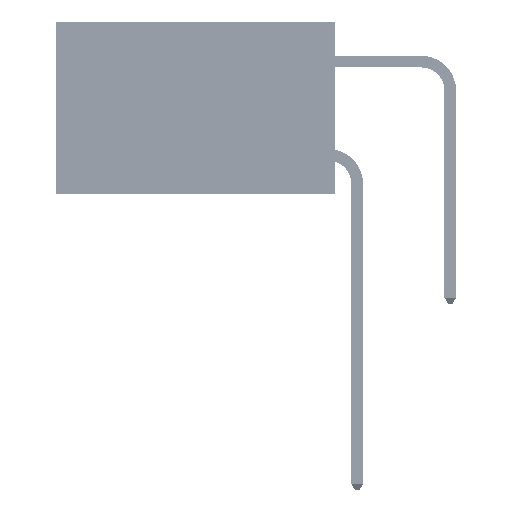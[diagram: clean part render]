
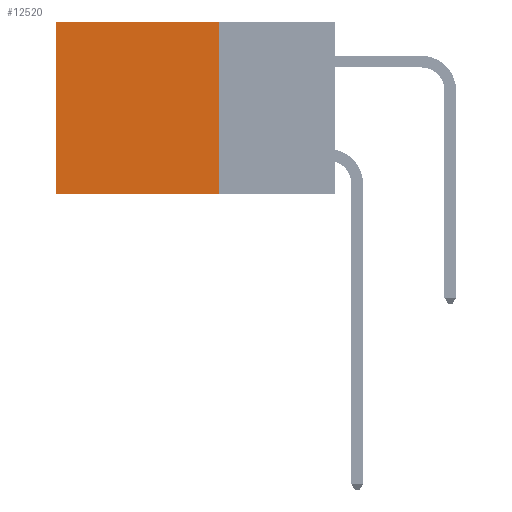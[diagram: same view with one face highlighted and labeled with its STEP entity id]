
A CAD part, left-side view. The second image highlights one B-rep face of the part: STEP entity #12520.
In plain terms, the highlighted planar face has unit normal (-1, 0, 0).
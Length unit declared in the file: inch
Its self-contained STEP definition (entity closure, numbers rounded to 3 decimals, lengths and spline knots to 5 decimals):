
#2174 = FACE_OUTER_BOUND ( 'NONE', #10021, .T. ) ;
#2588 = ORIENTED_EDGE ( 'NONE', *, *, #36556, .F. ) ;
#2835 = EDGE_CURVE ( 'NONE', #20938, #34990, #33069, .T. ) ;
#7108 = VECTOR ( 'NONE', #40612, 39.37008 ) ;
#7193 = VERTEX_POINT ( 'NONE', #37547 ) ;
#9708 = CARTESIAN_POINT ( 'NONE',  ( 0.2875, 0.25, 0. ) ) ;
#9715 = DIRECTION ( 'NONE',  ( 0., 0., -1. ) ) ;
#10021 = EDGE_LOOP ( 'NONE', ( #48256, #2588, #17914, #37603 ) ) ;
#10788 = LINE ( 'NONE', #20370, #15373 ) ;
#11294 = VERTEX_POINT ( 'NONE', #30142 ) ;
#11794 = CARTESIAN_POINT ( 'NONE',  ( 0.2875, 0.25, 0. ) ) ;
#12280 = EDGE_CURVE ( 'NONE', #20938, #7193, #10788, .T. ) ;
#12371 = CARTESIAN_POINT ( 'NONE',  ( 0.2875, 0.6, 0. ) ) ;
#12520 = ADVANCED_FACE ( 'NONE', ( #2174 ), #14109, .F. ) ;
#14109 = PLANE ( 'NONE',  #29498 ) ;
#15373 = VECTOR ( 'NONE', #32071, 39.37008 ) ;
#15978 = LINE ( 'NONE', #47431, #35932 ) ;
#17914 = ORIENTED_EDGE ( 'NONE', *, *, #12280, .F. ) ;
#20370 = CARTESIAN_POINT ( 'NONE',  ( 0.2875, 0.25, 0. ) ) ;
#20938 = VERTEX_POINT ( 'NONE', #11794 ) ;
#23981 = VECTOR ( 'NONE', #44082, 39.37008 ) ;
#26159 = CARTESIAN_POINT ( 'NONE',  ( 0.2875, 0.6, 0. ) ) ;
#27688 = DIRECTION ( 'NONE',  ( 0., 1., 0. ) ) ;
#29439 = CARTESIAN_POINT ( 'NONE',  ( 0.2875, 0.25, 0. ) ) ;
#29498 = AXIS2_PLACEMENT_3D ( 'NONE', #29439, #45302, #9715 ) ;
#30142 = CARTESIAN_POINT ( 'NONE',  ( 0.2875, 0.6, -0.37 ) ) ;
#32071 = DIRECTION ( 'NONE',  ( 0., 0., -1. ) ) ;
#32622 = LINE ( 'NONE', #12371, #23981 ) ;
#33069 = LINE ( 'NONE', #9708, #7108 ) ;
#34990 = VERTEX_POINT ( 'NONE', #26159 ) ;
#35932 = VECTOR ( 'NONE', #27688, 39.37008 ) ;
#36556 = EDGE_CURVE ( 'NONE', #7193, #11294, #15978, .T. ) ;
#37547 = CARTESIAN_POINT ( 'NONE',  ( 0.2875, 0.25, -0.37 ) ) ;
#37603 = ORIENTED_EDGE ( 'NONE', *, *, #2835, .T. ) ;
#40612 = DIRECTION ( 'NONE',  ( 0., 1., 0. ) ) ;
#44082 = DIRECTION ( 'NONE',  ( 0., 0., -1. ) ) ;
#45302 = DIRECTION ( 'NONE',  ( 1., 0., 0. ) ) ;
#46831 = EDGE_CURVE ( 'NONE', #34990, #11294, #32622, .T. ) ;
#47431 = CARTESIAN_POINT ( 'NONE',  ( 0.2875, 0.25, -0.37 ) ) ;
#48256 = ORIENTED_EDGE ( 'NONE', *, *, #46831, .T. ) ;
